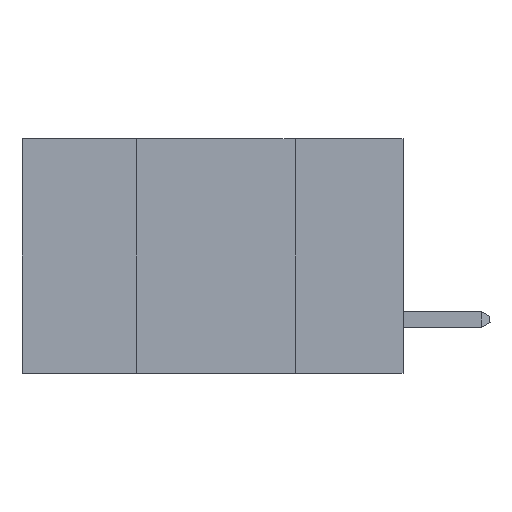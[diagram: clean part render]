
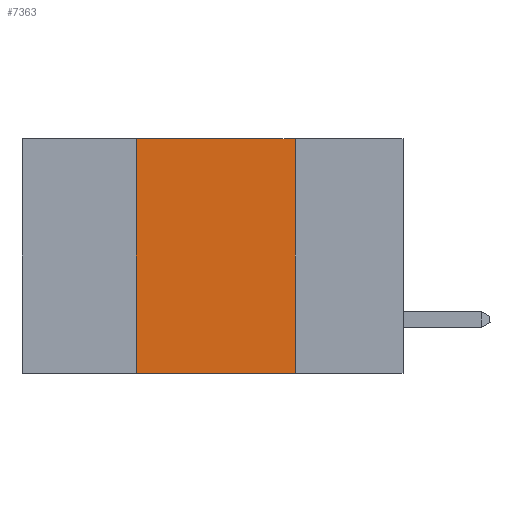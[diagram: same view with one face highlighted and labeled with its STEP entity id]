
A CAD part, left-side view. The second image highlights one B-rep face of the part: STEP entity #7363.
In plain terms, the highlighted planar face has unit normal (-1, 0, 0).
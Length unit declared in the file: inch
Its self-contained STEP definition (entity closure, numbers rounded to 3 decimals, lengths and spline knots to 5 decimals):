
#502 = LINE ( 'NONE', #3632, #8242 ) ;
#555 = LINE ( 'NONE', #2265, #12606 ) ;
#1899 = VERTEX_POINT ( 'NONE', #3794 ) ;
#2265 = CARTESIAN_POINT ( 'NONE',  ( 0., 0.6, -0.37 ) ) ;
#2287 = LINE ( 'NONE', #4714, #17744 ) ;
#2319 = LINE ( 'NONE', #9195, #14383 ) ;
#2415 = DIRECTION ( 'NONE',  ( 0., -1., 0. ) ) ;
#3412 = CARTESIAN_POINT ( 'NONE',  ( 0., 0.42, 0. ) ) ;
#3590 = EDGE_LOOP ( 'NONE', ( #14213, #19518, #3995, #3937 ) ) ;
#3632 = CARTESIAN_POINT ( 'NONE',  ( 0., 0.42, 0. ) ) ;
#3794 = CARTESIAN_POINT ( 'NONE',  ( 0., 0.42, -0.37 ) ) ;
#3937 = ORIENTED_EDGE ( 'NONE', *, *, #17648, .T. ) ;
#3963 = EDGE_CURVE ( 'NONE', #17898, #8489, #2287, .T. ) ;
#3995 = ORIENTED_EDGE ( 'NONE', *, *, #10739, .F. ) ;
#4635 = PLANE ( 'NONE',  #17759 ) ;
#4714 = CARTESIAN_POINT ( 'NONE',  ( 0., 0.17, 0. ) ) ;
#4848 = EDGE_CURVE ( 'NONE', #18321, #17898, #2319, .T. ) ;
#5159 = DIRECTION ( 'NONE',  ( 1., 0., 0. ) ) ;
#7363 = ADVANCED_FACE ( 'NONE', ( #15495 ), #4635, .F. ) ;
#8242 = VECTOR ( 'NONE', #19182, 39.37008 ) ;
#8489 = VERTEX_POINT ( 'NONE', #16283 ) ;
#9195 = CARTESIAN_POINT ( 'NONE',  ( 0., 0.6, 0. ) ) ;
#10739 = EDGE_CURVE ( 'NONE', #1899, #18321, #502, .T. ) ;
#12606 = VECTOR ( 'NONE', #13074, 39.37008 ) ;
#13074 = DIRECTION ( 'NONE',  ( 0., -1., 0. ) ) ;
#14213 = ORIENTED_EDGE ( 'NONE', *, *, #3963, .F. ) ;
#14286 = DIRECTION ( 'NONE',  ( 0., 0., -1. ) ) ;
#14383 = VECTOR ( 'NONE', #2415, 39.37008 ) ;
#15469 = DIRECTION ( 'NONE',  ( 0., 0., -1. ) ) ;
#15495 = FACE_OUTER_BOUND ( 'NONE', #3590, .T. ) ;
#15772 = CARTESIAN_POINT ( 'NONE',  ( 0., 0.6, 0. ) ) ;
#16283 = CARTESIAN_POINT ( 'NONE',  ( 0., 0.17, -0.37 ) ) ;
#16807 = CARTESIAN_POINT ( 'NONE',  ( 0., 0.17, 0. ) ) ;
#17648 = EDGE_CURVE ( 'NONE', #1899, #8489, #555, .T. ) ;
#17744 = VECTOR ( 'NONE', #15469, 39.37008 ) ;
#17759 = AXIS2_PLACEMENT_3D ( 'NONE', #15772, #5159, #14286 ) ;
#17898 = VERTEX_POINT ( 'NONE', #16807 ) ;
#18321 = VERTEX_POINT ( 'NONE', #3412 ) ;
#19182 = DIRECTION ( 'NONE',  ( 0., 0., 1. ) ) ;
#19518 = ORIENTED_EDGE ( 'NONE', *, *, #4848, .F. ) ;
